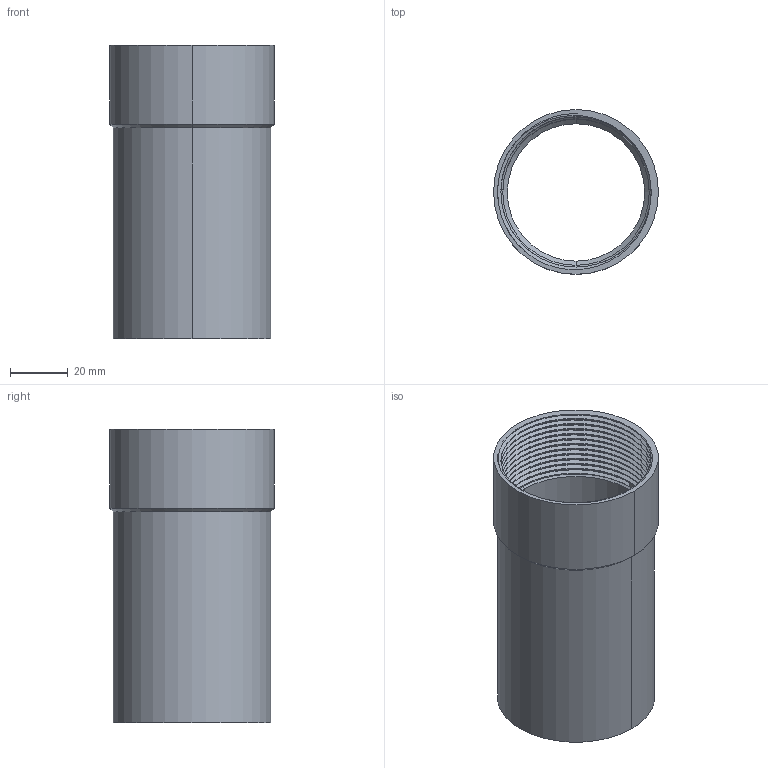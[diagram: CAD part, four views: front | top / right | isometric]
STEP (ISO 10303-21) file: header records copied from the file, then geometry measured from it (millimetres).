
FILE_DESCRIPTION (( 'STEP AP203' ), '1' );
FILE_NAME ('AF-22LRPP-SB-PRT-002-STEP.STEP', '2020-08-30T06:47:49', ( '' ), ( '' ), 'SwSTEP 2.0', 'SolidWorks 2018', '' );
FILE_SCHEMA (( 'CONFIG_CONTROL_DESIGN' ));
Length unit declared in the file: inch
Products named in the file (1): AF-22LRPP-SB-PRT-002-STEP
Bounding box: 57.15 x 57.15 x 101.6 mm (x, y, z)
Volume: 34371.5 mm3; surface area: 37700.2 mm2
Topology: 1 solids, 1 shells, 45 faces, 115 edges, 72 vertices
Faces by surface type: cylinder 33, cone 6, plane 3, bspline 3
Entity records: 3810 total; most frequent: CARTESIAN_POINT 2791, ORIENTED_EDGE 230, DIRECTION 168, EDGE_CURVE 115, VERTEX_POINT 72, AXIS2_PLACEMENT_3D 63, EDGE_LOOP 47, ADVANCED_FACE 45
